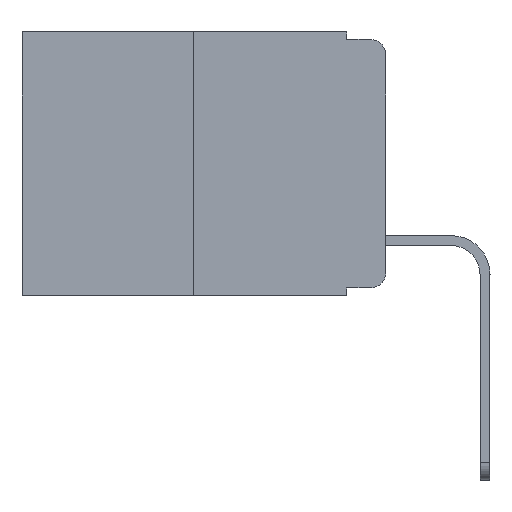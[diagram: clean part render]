
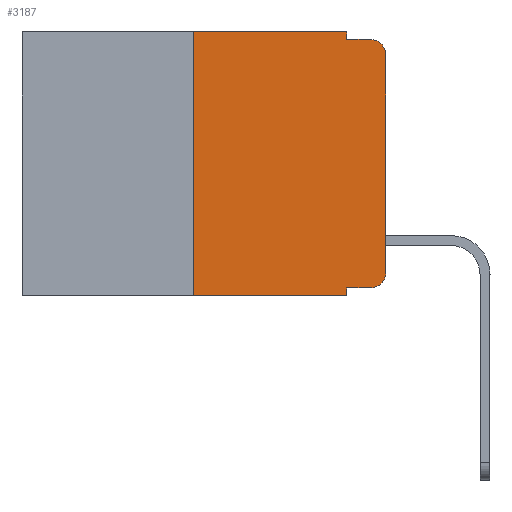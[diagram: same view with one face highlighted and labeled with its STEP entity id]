
A CAD part, left-side view. The second image highlights one B-rep face of the part: STEP entity #3187.
In plain terms, the highlighted planar face has unit normal (-1, 0, 0).
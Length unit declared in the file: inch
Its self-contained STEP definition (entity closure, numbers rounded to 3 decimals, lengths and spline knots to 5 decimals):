
#347 = ORIENTED_EDGE ( 'NONE', *, *, #10260, .T. ) ;
#385 = ORIENTED_EDGE ( 'NONE', *, *, #3923, .F. ) ;
#738 = CARTESIAN_POINT ( 'NONE',  ( 0., 0.473, -0.343 ) ) ;
#905 = ORIENTED_EDGE ( 'NONE', *, *, #3301, .T. ) ;
#1391 = CARTESIAN_POINT ( 'NONE',  ( 0., 0.051, -0.333 ) ) ;
#1886 = CIRCLE ( 'NONE', #18488, 0.02 ) ;
#1907 = VECTOR ( 'NONE', #7420, 39.37008 ) ;
#1969 = CARTESIAN_POINT ( 'NONE',  ( 0., 0., -0.03 ) ) ;
#2152 = ORIENTED_EDGE ( 'NONE', *, *, #9348, .T. ) ;
#2163 = CARTESIAN_POINT ( 'NONE',  ( 0., 0., -0.313 ) ) ;
#2348 = CIRCLE ( 'NONE', #20389, 0.02 ) ;
#2697 = CARTESIAN_POINT ( 'NONE',  ( 0., 0.25, 0. ) ) ;
#2785 = VERTEX_POINT ( 'NONE', #20590 ) ;
#3187 = ADVANCED_FACE ( 'NONE', ( #10962 ), #11918, .F. ) ;
#3207 = VERTEX_POINT ( 'NONE', #5242 ) ;
#3301 = EDGE_CURVE ( 'NONE', #12202, #10807, #20617, .T. ) ;
#3579 = LINE ( 'NONE', #6314, #13062 ) ;
#3734 = LINE ( 'NONE', #17303, #9651 ) ;
#3793 = VECTOR ( 'NONE', #12279, 39.37008 ) ;
#3865 = DIRECTION ( 'NONE',  ( 0., 0., -1. ) ) ;
#3923 = EDGE_CURVE ( 'NONE', #12202, #2785, #7349, .T. ) ;
#4532 = DIRECTION ( 'NONE',  ( 0., 0., -1. ) ) ;
#4667 = CARTESIAN_POINT ( 'NONE',  ( 0., 0.02, -0.313 ) ) ;
#5242 = CARTESIAN_POINT ( 'NONE',  ( 0., 0.051, 0. ) ) ;
#5356 = EDGE_CURVE ( 'NONE', #8017, #17156, #9177, .T. ) ;
#5370 = DIRECTION ( 'NONE',  ( 0., -1., 0. ) ) ;
#6314 = CARTESIAN_POINT ( 'NONE',  ( 0., 0., 0. ) ) ;
#6410 = CARTESIAN_POINT ( 'NONE',  ( 0., 0.051, -0.01 ) ) ;
#7073 = VERTEX_POINT ( 'NONE', #1969 ) ;
#7349 = LINE ( 'NONE', #2697, #15529 ) ;
#7420 = DIRECTION ( 'NONE',  ( 0., -1., 0. ) ) ;
#7435 = DIRECTION ( 'NONE',  ( 0., 0., 1. ) ) ;
#7839 = ORIENTED_EDGE ( 'NONE', *, *, #17684, .F. ) ;
#8017 = VERTEX_POINT ( 'NONE', #1391 ) ;
#8628 = CARTESIAN_POINT ( 'NONE',  ( 0., 0.051, -0.333 ) ) ;
#8911 = ORIENTED_EDGE ( 'NONE', *, *, #11790, .F. ) ;
#8918 = ORIENTED_EDGE ( 'NONE', *, *, #16683, .T. ) ;
#9177 = LINE ( 'NONE', #8628, #9933 ) ;
#9182 = DIRECTION ( 'NONE',  ( 0., 0., -1. ) ) ;
#9348 = EDGE_CURVE ( 'NONE', #17156, #19408, #2348, .T. ) ;
#9453 = VERTEX_POINT ( 'NONE', #14633 ) ;
#9651 = VECTOR ( 'NONE', #9182, 39.37008 ) ;
#9933 = VECTOR ( 'NONE', #10268, 39.37008 ) ;
#10260 = EDGE_CURVE ( 'NONE', #7073, #9453, #1886, .T. ) ;
#10268 = DIRECTION ( 'NONE',  ( 0., -1., 0. ) ) ;
#10626 = CARTESIAN_POINT ( 'NONE',  ( 0., 0.051, 0. ) ) ;
#10807 = VERTEX_POINT ( 'NONE', #15409 ) ;
#10830 = EDGE_CURVE ( 'NONE', #8017, #10807, #18611, .T. ) ;
#10924 = CARTESIAN_POINT ( 'NONE',  ( 0., 0.02, -0.333 ) ) ;
#10940 = VECTOR ( 'NONE', #12194, 39.37008 ) ;
#10962 = FACE_OUTER_BOUND ( 'NONE', #11726, .T. ) ;
#11726 = EDGE_LOOP ( 'NONE', ( #8918, #347, #12996, #7839, #8911, #385, #905, #18670, #15712, #2152 ) ) ;
#11790 = EDGE_CURVE ( 'NONE', #2785, #3207, #18297, .T. ) ;
#11918 = PLANE ( 'NONE',  #19883 ) ;
#11987 = DIRECTION ( 'NONE',  ( 1., 0., 0. ) ) ;
#12071 = DIRECTION ( 'NONE',  ( 0., 0., 1. ) ) ;
#12194 = DIRECTION ( 'NONE',  ( 0., -1., 0. ) ) ;
#12202 = VERTEX_POINT ( 'NONE', #20976 ) ;
#12279 = DIRECTION ( 'NONE',  ( 0., 0., -1. ) ) ;
#12803 = VERTEX_POINT ( 'NONE', #6410 ) ;
#12996 = ORIENTED_EDGE ( 'NONE', *, *, #14038, .F. ) ;
#13062 = VECTOR ( 'NONE', #12071, 39.37008 ) ;
#14038 = EDGE_CURVE ( 'NONE', #12803, #9453, #14956, .T. ) ;
#14517 = VECTOR ( 'NONE', #5370, 39.37008 ) ;
#14633 = CARTESIAN_POINT ( 'NONE',  ( 0., 0.02, -0.01 ) ) ;
#14956 = LINE ( 'NONE', #20600, #1907 ) ;
#15409 = CARTESIAN_POINT ( 'NONE',  ( 0., 0.051, -0.343 ) ) ;
#15449 = CARTESIAN_POINT ( 'NONE',  ( 0., 0.02, -0.03 ) ) ;
#15525 = DIRECTION ( 'NONE',  ( -1., 0., 0. ) ) ;
#15529 = VECTOR ( 'NONE', #7435, 39.37008 ) ;
#15712 = ORIENTED_EDGE ( 'NONE', *, *, #5356, .T. ) ;
#16683 = EDGE_CURVE ( 'NONE', #19408, #7073, #3579, .T. ) ;
#16929 = CARTESIAN_POINT ( 'NONE',  ( 0., 0.473, 0. ) ) ;
#17141 = DIRECTION ( 'NONE',  ( 0., 0., -1. ) ) ;
#17156 = VERTEX_POINT ( 'NONE', #10924 ) ;
#17303 = CARTESIAN_POINT ( 'NONE',  ( 0., 0.051, 0. ) ) ;
#17684 = EDGE_CURVE ( 'NONE', #3207, #12803, #3734, .T. ) ;
#18297 = LINE ( 'NONE', #16929, #14517 ) ;
#18488 = AXIS2_PLACEMENT_3D ( 'NONE', #15449, #15525, #17141 ) ;
#18611 = LINE ( 'NONE', #10626, #3793 ) ;
#18670 = ORIENTED_EDGE ( 'NONE', *, *, #10830, .F. ) ;
#19378 = DIRECTION ( 'NONE',  ( -1., 0., 0. ) ) ;
#19408 = VERTEX_POINT ( 'NONE', #2163 ) ;
#19860 = CARTESIAN_POINT ( 'NONE',  ( 0., 0.473, 0. ) ) ;
#19883 = AXIS2_PLACEMENT_3D ( 'NONE', #19860, #11987, #3865 ) ;
#20389 = AXIS2_PLACEMENT_3D ( 'NONE', #4667, #19378, #4532 ) ;
#20590 = CARTESIAN_POINT ( 'NONE',  ( 0., 0.25, 0. ) ) ;
#20600 = CARTESIAN_POINT ( 'NONE',  ( 0., 0.051, -0.01 ) ) ;
#20617 = LINE ( 'NONE', #738, #10940 ) ;
#20976 = CARTESIAN_POINT ( 'NONE',  ( 0., 0.25, -0.343 ) ) ;
